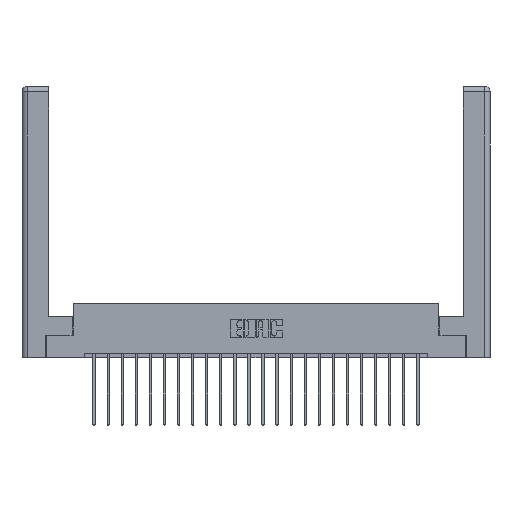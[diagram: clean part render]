
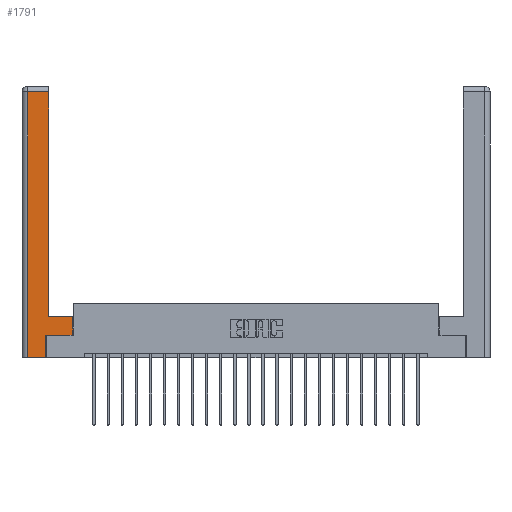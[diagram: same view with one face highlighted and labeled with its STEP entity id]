
A CAD part, top view. The second image highlights one B-rep face of the part: STEP entity #1791.
In plain terms, the highlighted planar face has unit normal (0, 0, 1).
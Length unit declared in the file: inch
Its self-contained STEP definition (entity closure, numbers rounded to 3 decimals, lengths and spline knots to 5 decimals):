
#338 = VECTOR ( 'NONE', #8559, 39.37008 ) ;
#492 = CARTESIAN_POINT ( 'NONE',  ( 0.0615, 0., 0. ) ) ;
#657 = ORIENTED_EDGE ( 'NONE', *, *, #7378, .T. ) ;
#1167 = LINE ( 'NONE', #3101, #12008 ) ;
#1738 = EDGE_CURVE ( 'NONE', #2815, #17748, #19109, .T. ) ;
#1758 = LINE ( 'NONE', #21238, #338 ) ;
#1791 = ADVANCED_FACE ( 'NONE', ( #3156 ), #2410, .F. ) ;
#1947 = EDGE_CURVE ( 'NONE', #19829, #2815, #1758, .T. ) ;
#1968 = CARTESIAN_POINT ( 'NONE',  ( 0.565, 0.245, 0. ) ) ;
#2169 = DIRECTION ( 'NONE',  ( 1., 0., 0. ) ) ;
#2187 = EDGE_CURVE ( 'NONE', #17748, #4200, #1167, .T. ) ;
#2252 = CARTESIAN_POINT ( 'NONE',  ( 0.265, 0., 0. ) ) ;
#2353 = AXIS2_PLACEMENT_3D ( 'NONE', #6090, #4320, #15251 ) ;
#2410 = PLANE ( 'NONE',  #2353 ) ;
#2815 = VERTEX_POINT ( 'NONE', #10203 ) ;
#3101 = CARTESIAN_POINT ( 'NONE',  ( 0.565, 0.45, 0. ) ) ;
#3156 = FACE_OUTER_BOUND ( 'NONE', #15890, .T. ) ;
#3174 = ORIENTED_EDGE ( 'NONE', *, *, #6777, .T. ) ;
#3422 = CARTESIAN_POINT ( 'NONE',  ( 0.565, 0.45, 0. ) ) ;
#3579 = LINE ( 'NONE', #16344, #18706 ) ;
#4200 = VERTEX_POINT ( 'NONE', #3422 ) ;
#4320 = DIRECTION ( 'NONE',  ( 0., 0., -1. ) ) ;
#4458 = ORIENTED_EDGE ( 'NONE', *, *, #21681, .T. ) ;
#6090 = CARTESIAN_POINT ( 'NONE',  ( 0., 0., 0. ) ) ;
#6747 = VECTOR ( 'NONE', #15429, 39.37008 ) ;
#6777 = EDGE_CURVE ( 'NONE', #4200, #19684, #3579, .T. ) ;
#7009 = ORIENTED_EDGE ( 'NONE', *, *, #1947, .T. ) ;
#7228 = VECTOR ( 'NONE', #10395, 39.37008 ) ;
#7378 = EDGE_CURVE ( 'NONE', #22394, #13382, #7876, .T. ) ;
#7663 = ORIENTED_EDGE ( 'NONE', *, *, #19570, .T. ) ;
#7876 = LINE ( 'NONE', #9939, #6747 ) ;
#7882 = ORIENTED_EDGE ( 'NONE', *, *, #1738, .T. ) ;
#8559 = DIRECTION ( 'NONE',  ( 0., 1., 0. ) ) ;
#9432 = CARTESIAN_POINT ( 'NONE',  ( 0.295, 0.45, 0. ) ) ;
#9485 = EDGE_CURVE ( 'NONE', #13382, #19829, #17177, .T. ) ;
#9654 = DIRECTION ( 'NONE',  ( 1., 0., 0. ) ) ;
#9939 = CARTESIAN_POINT ( 'NONE',  ( 0.0615, 0., 0. ) ) ;
#9974 = DIRECTION ( 'NONE',  ( -1., 0., 0. ) ) ;
#10203 = CARTESIAN_POINT ( 'NONE',  ( 0.265, 0.245, 0. ) ) ;
#10323 = CARTESIAN_POINT ( 'NONE',  ( 0.295, 3., 0. ) ) ;
#10395 = DIRECTION ( 'NONE',  ( 0., 1., 0. ) ) ;
#12008 = VECTOR ( 'NONE', #13840, 39.37008 ) ;
#13311 = CARTESIAN_POINT ( 'NONE',  ( 0.265, 0., 0. ) ) ;
#13382 = VERTEX_POINT ( 'NONE', #492 ) ;
#13840 = DIRECTION ( 'NONE',  ( 0., 1., 0. ) ) ;
#14421 = DIRECTION ( 'NONE',  ( -1., 0., 0. ) ) ;
#15101 = VECTOR ( 'NONE', #9974, 39.37008 ) ;
#15251 = DIRECTION ( 'NONE',  ( -1., 0., 0. ) ) ;
#15429 = DIRECTION ( 'NONE',  ( 0., -1., 0. ) ) ;
#15890 = EDGE_LOOP ( 'NONE', ( #7663, #4458, #657, #18131, #7009, #7882, #21294, #3174 ) ) ;
#16169 = CARTESIAN_POINT ( 'NONE',  ( 0.0615, 2.94, 0. ) ) ;
#16344 = CARTESIAN_POINT ( 'NONE',  ( 0.295, 0.45, 0. ) ) ;
#16819 = VECTOR ( 'NONE', #9654, 39.37008 ) ;
#17093 = LINE ( 'NONE', #19049, #15101 ) ;
#17177 = LINE ( 'NONE', #2252, #18304 ) ;
#17748 = VERTEX_POINT ( 'NONE', #1968 ) ;
#18040 = LINE ( 'NONE', #10323, #7228 ) ;
#18131 = ORIENTED_EDGE ( 'NONE', *, *, #9485, .T. ) ;
#18304 = VECTOR ( 'NONE', #2169, 39.37008 ) ;
#18706 = VECTOR ( 'NONE', #14421, 39.37008 ) ;
#19049 = CARTESIAN_POINT ( 'NONE',  ( 0.0615, 2.94, 0. ) ) ;
#19109 = LINE ( 'NONE', #20653, #16819 ) ;
#19521 = CARTESIAN_POINT ( 'NONE',  ( 0.295, 2.94, 0. ) ) ;
#19570 = EDGE_CURVE ( 'NONE', #19684, #21345, #18040, .T. ) ;
#19684 = VERTEX_POINT ( 'NONE', #9432 ) ;
#19829 = VERTEX_POINT ( 'NONE', #13311 ) ;
#20653 = CARTESIAN_POINT ( 'NONE',  ( 0.565, 0.245, 0. ) ) ;
#21238 = CARTESIAN_POINT ( 'NONE',  ( 0.265, 0.245, 0. ) ) ;
#21294 = ORIENTED_EDGE ( 'NONE', *, *, #2187, .T. ) ;
#21345 = VERTEX_POINT ( 'NONE', #19521 ) ;
#21681 = EDGE_CURVE ( 'NONE', #21345, #22394, #17093, .T. ) ;
#22394 = VERTEX_POINT ( 'NONE', #16169 ) ;
